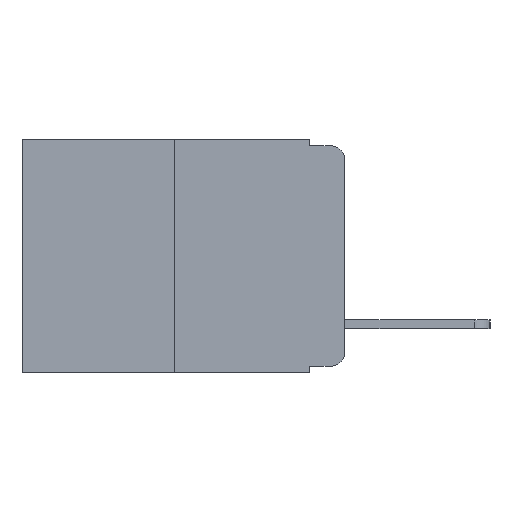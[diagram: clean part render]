
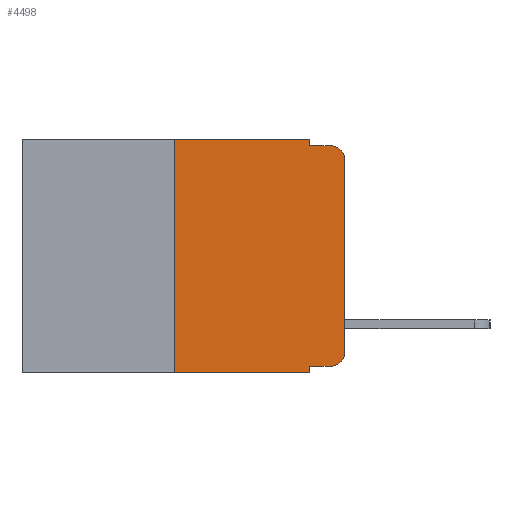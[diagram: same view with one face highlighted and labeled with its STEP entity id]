
A CAD part, left-side view. The second image highlights one B-rep face of the part: STEP entity #4498.
In plain terms, the highlighted planar face has unit normal (-1, 0, 0).
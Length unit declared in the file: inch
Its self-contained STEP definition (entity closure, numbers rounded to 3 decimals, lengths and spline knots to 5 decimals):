
#86 = CARTESIAN_POINT ( 'NONE',  ( 0., 0.02, -0.01 ) ) ;
#182 = VERTEX_POINT ( 'NONE', #2337 ) ;
#227 = CARTESIAN_POINT ( 'NONE',  ( 0., 0.051, -0.343 ) ) ;
#274 = LINE ( 'NONE', #10451, #5393 ) ;
#294 = CIRCLE ( 'NONE', #5235, 0.02 ) ;
#606 = CARTESIAN_POINT ( 'NONE',  ( 0., 0.051, 0. ) ) ;
#1049 = LINE ( 'NONE', #606, #6330 ) ;
#1293 = ORIENTED_EDGE ( 'NONE', *, *, #6052, .T. ) ;
#1367 = DIRECTION ( 'NONE',  ( 0., 0., -1. ) ) ;
#1569 = CARTESIAN_POINT ( 'NONE',  ( 0., 0., -0.313 ) ) ;
#1691 = VERTEX_POINT ( 'NONE', #4107 ) ;
#1700 = ORIENTED_EDGE ( 'NONE', *, *, #6495, .F. ) ;
#1717 = ORIENTED_EDGE ( 'NONE', *, *, #5304, .F. ) ;
#1726 = DIRECTION ( 'NONE',  ( 0., -1., 0. ) ) ;
#1858 = AXIS2_PLACEMENT_3D ( 'NONE', #10173, #5238, #10941 ) ;
#1873 = ORIENTED_EDGE ( 'NONE', *, *, #6348, .F. ) ;
#2036 = EDGE_LOOP ( 'NONE', ( #1293, #7936, #1873, #2772, #1717, #1700, #3375, #3414, #3938, #9246 ) ) ;
#2114 = CARTESIAN_POINT ( 'NONE',  ( 0., 0.25, -0.343 ) ) ;
#2337 = CARTESIAN_POINT ( 'NONE',  ( 0., 0.25, 0. ) ) ;
#2772 = ORIENTED_EDGE ( 'NONE', *, *, #6416, .F. ) ;
#3056 = VERTEX_POINT ( 'NONE', #2114 ) ;
#3060 = VECTOR ( 'NONE', #4829, 39.37008 ) ;
#3108 = VERTEX_POINT ( 'NONE', #1569 ) ;
#3169 = DIRECTION ( 'NONE',  ( 0., -1., 0. ) ) ;
#3317 = VECTOR ( 'NONE', #3169, 39.37008 ) ;
#3375 = ORIENTED_EDGE ( 'NONE', *, *, #6571, .T. ) ;
#3391 = LINE ( 'NONE', #6768, #7809 ) ;
#3414 = ORIENTED_EDGE ( 'NONE', *, *, #7305, .F. ) ;
#3938 = ORIENTED_EDGE ( 'NONE', *, *, #8187, .T. ) ;
#4107 = CARTESIAN_POINT ( 'NONE',  ( 0., 0., -0.03 ) ) ;
#4108 = CARTESIAN_POINT ( 'NONE',  ( 0., 0.02, -0.03 ) ) ;
#4140 = AXIS2_PLACEMENT_3D ( 'NONE', #10336, #8242, #8802 ) ;
#4220 = CARTESIAN_POINT ( 'NONE',  ( 0., 0.051, -0.01 ) ) ;
#4498 = ADVANCED_FACE ( 'NONE', ( #8449 ), #7026, .F. ) ;
#4532 = LINE ( 'NONE', #6820, #8545 ) ;
#4829 = DIRECTION ( 'NONE',  ( 0., -1., 0. ) ) ;
#5235 = AXIS2_PLACEMENT_3D ( 'NONE', #4108, #9393, #9382 ) ;
#5238 = DIRECTION ( 'NONE',  ( -1., 0., 0. ) ) ;
#5304 = EDGE_CURVE ( 'NONE', #182, #9109, #6629, .T. ) ;
#5393 = VECTOR ( 'NONE', #8346, 39.37008 ) ;
#5540 = LINE ( 'NONE', #4220, #3060 ) ;
#6052 = EDGE_CURVE ( 'NONE', #3108, #1691, #3391, .T. ) ;
#6179 = VERTEX_POINT ( 'NONE', #6347 ) ;
#6221 = EDGE_CURVE ( 'NONE', #1691, #6568, #294, .T. ) ;
#6262 = DIRECTION ( 'NONE',  ( 0., 0., -1. ) ) ;
#6330 = VECTOR ( 'NONE', #6262, 39.37008 ) ;
#6347 = CARTESIAN_POINT ( 'NONE',  ( 0., 0.02, -0.333 ) ) ;
#6348 = EDGE_CURVE ( 'NONE', #7383, #6568, #5540, .T. ) ;
#6416 = EDGE_CURVE ( 'NONE', #9109, #7383, #8689, .T. ) ;
#6421 = VERTEX_POINT ( 'NONE', #8753 ) ;
#6495 = EDGE_CURVE ( 'NONE', #3056, #182, #274, .T. ) ;
#6568 = VERTEX_POINT ( 'NONE', #86 ) ;
#6571 = EDGE_CURVE ( 'NONE', #3056, #8206, #4532, .T. ) ;
#6629 = LINE ( 'NONE', #7542, #10631 ) ;
#6768 = CARTESIAN_POINT ( 'NONE',  ( 0., 0., 0. ) ) ;
#6820 = CARTESIAN_POINT ( 'NONE',  ( 0., 0.473, -0.343 ) ) ;
#7026 = PLANE ( 'NONE',  #4140 ) ;
#7116 = DIRECTION ( 'NONE',  ( 0., 0., 1. ) ) ;
#7256 = CIRCLE ( 'NONE', #1858, 0.02 ) ;
#7257 = CARTESIAN_POINT ( 'NONE',  ( 0., 0.051, -0.01 ) ) ;
#7305 = EDGE_CURVE ( 'NONE', #6421, #8206, #1049, .T. ) ;
#7383 = VERTEX_POINT ( 'NONE', #7257 ) ;
#7542 = CARTESIAN_POINT ( 'NONE',  ( 0., 0.473, 0. ) ) ;
#7809 = VECTOR ( 'NONE', #7116, 39.37008 ) ;
#7936 = ORIENTED_EDGE ( 'NONE', *, *, #6221, .T. ) ;
#8187 = EDGE_CURVE ( 'NONE', #6421, #6179, #10106, .T. ) ;
#8206 = VERTEX_POINT ( 'NONE', #227 ) ;
#8242 = DIRECTION ( 'NONE',  ( 1., 0., 0. ) ) ;
#8295 = EDGE_CURVE ( 'NONE', #6179, #3108, #7256, .T. ) ;
#8346 = DIRECTION ( 'NONE',  ( 0., 0., 1. ) ) ;
#8449 = FACE_OUTER_BOUND ( 'NONE', #2036, .T. ) ;
#8545 = VECTOR ( 'NONE', #9182, 39.37008 ) ;
#8689 = LINE ( 'NONE', #8766, #11210 ) ;
#8753 = CARTESIAN_POINT ( 'NONE',  ( 0., 0.051, -0.333 ) ) ;
#8766 = CARTESIAN_POINT ( 'NONE',  ( 0., 0.051, 0. ) ) ;
#8802 = DIRECTION ( 'NONE',  ( 0., 0., -1. ) ) ;
#9109 = VERTEX_POINT ( 'NONE', #10597 ) ;
#9182 = DIRECTION ( 'NONE',  ( 0., -1., 0. ) ) ;
#9246 = ORIENTED_EDGE ( 'NONE', *, *, #8295, .T. ) ;
#9382 = DIRECTION ( 'NONE',  ( 0., 0., -1. ) ) ;
#9393 = DIRECTION ( 'NONE',  ( -1., 0., 0. ) ) ;
#10106 = LINE ( 'NONE', #10773, #3317 ) ;
#10173 = CARTESIAN_POINT ( 'NONE',  ( 0., 0.02, -0.313 ) ) ;
#10336 = CARTESIAN_POINT ( 'NONE',  ( 0., 0.473, 0. ) ) ;
#10451 = CARTESIAN_POINT ( 'NONE',  ( 0., 0.25, 0. ) ) ;
#10597 = CARTESIAN_POINT ( 'NONE',  ( 0., 0.051, 0. ) ) ;
#10631 = VECTOR ( 'NONE', #1726, 39.37008 ) ;
#10773 = CARTESIAN_POINT ( 'NONE',  ( 0., 0.051, -0.333 ) ) ;
#10941 = DIRECTION ( 'NONE',  ( 0., 0., -1. ) ) ;
#11210 = VECTOR ( 'NONE', #1367, 39.37008 ) ;
